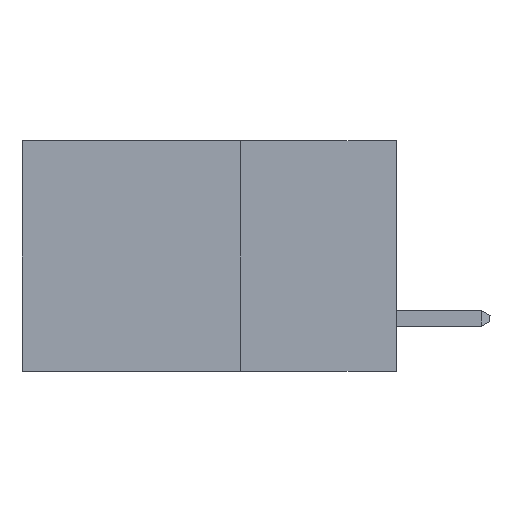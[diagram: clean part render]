
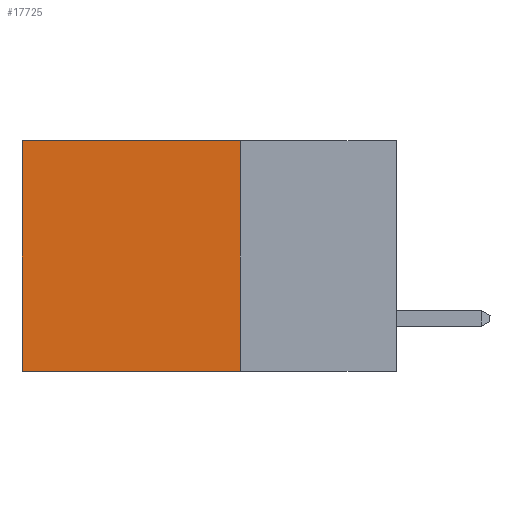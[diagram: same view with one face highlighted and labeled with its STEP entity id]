
A CAD part, left-side view. The second image highlights one B-rep face of the part: STEP entity #17725.
In plain terms, the highlighted planar face has unit normal (-1, 0, 0).
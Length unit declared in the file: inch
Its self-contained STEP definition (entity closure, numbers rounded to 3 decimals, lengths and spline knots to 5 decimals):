
#540 = LINE ( 'NONE', #2983, #13661 ) ;
#1282 = ORIENTED_EDGE ( 'NONE', *, *, #10038, .F. ) ;
#1720 = ORIENTED_EDGE ( 'NONE', *, *, #2895, .F. ) ;
#2859 = DIRECTION ( 'NONE',  ( 0., 1., 0. ) ) ;
#2895 = EDGE_CURVE ( 'NONE', #9882, #13582, #540, .T. ) ;
#2983 = CARTESIAN_POINT ( 'NONE',  ( 0.2615, 0.25, -0.37 ) ) ;
#3314 = ORIENTED_EDGE ( 'NONE', *, *, #23565, .T. ) ;
#3834 = DIRECTION ( 'NONE',  ( 0., 0., -1. ) ) ;
#4135 = DIRECTION ( 'NONE',  ( 0., 0., -1. ) ) ;
#5768 = CARTESIAN_POINT ( 'NONE',  ( 0.2615, 0.25, -0.37 ) ) ;
#9542 = FACE_OUTER_BOUND ( 'NONE', #9607, .T. ) ;
#9545 = DIRECTION ( 'NONE',  ( 0., 0., -1. ) ) ;
#9571 = CARTESIAN_POINT ( 'NONE',  ( 0.2615, 0.6, -0.37 ) ) ;
#9607 = EDGE_LOOP ( 'NONE', ( #11316, #1282, #1720, #3314 ) ) ;
#9851 = CARTESIAN_POINT ( 'NONE',  ( 0.2615, 0.25, -0.37 ) ) ;
#9882 = VERTEX_POINT ( 'NONE', #13881 ) ;
#10038 = EDGE_CURVE ( 'NONE', #13582, #10863, #15466, .T. ) ;
#10395 = VECTOR ( 'NONE', #22496, 39.37008 ) ;
#10863 = VERTEX_POINT ( 'NONE', #13765 ) ;
#11316 = ORIENTED_EDGE ( 'NONE', *, *, #13600, .T. ) ;
#11406 = VECTOR ( 'NONE', #9545, 39.37008 ) ;
#11490 = PLANE ( 'NONE',  #22700 ) ;
#11701 = VECTOR ( 'NONE', #2859, 39.37008 ) ;
#11985 = LINE ( 'NONE', #9571, #11406 ) ;
#12945 = VERTEX_POINT ( 'NONE', #16747 ) ;
#13398 = CARTESIAN_POINT ( 'NONE',  ( 0.2615, 0.25, -0.37 ) ) ;
#13582 = VERTEX_POINT ( 'NONE', #9851 ) ;
#13600 = EDGE_CURVE ( 'NONE', #12945, #10863, #11985, .T. ) ;
#13661 = VECTOR ( 'NONE', #3834, 39.37008 ) ;
#13765 = CARTESIAN_POINT ( 'NONE',  ( 0.2615, 0.6, -0.37 ) ) ;
#13881 = CARTESIAN_POINT ( 'NONE',  ( 0.2615, 0.25, 0. ) ) ;
#15315 = DIRECTION ( 'NONE',  ( 1., 0., 0. ) ) ;
#15466 = LINE ( 'NONE', #5768, #10395 ) ;
#16747 = CARTESIAN_POINT ( 'NONE',  ( 0.2615, 0.6, 0. ) ) ;
#17725 = ADVANCED_FACE ( 'NONE', ( #9542 ), #11490, .F. ) ;
#19540 = CARTESIAN_POINT ( 'NONE',  ( 0.2615, 0.25, 0. ) ) ;
#22017 = LINE ( 'NONE', #19540, #11701 ) ;
#22496 = DIRECTION ( 'NONE',  ( 0., 1., 0. ) ) ;
#22700 = AXIS2_PLACEMENT_3D ( 'NONE', #13398, #15315, #4135 ) ;
#23565 = EDGE_CURVE ( 'NONE', #9882, #12945, #22017, .T. ) ;
